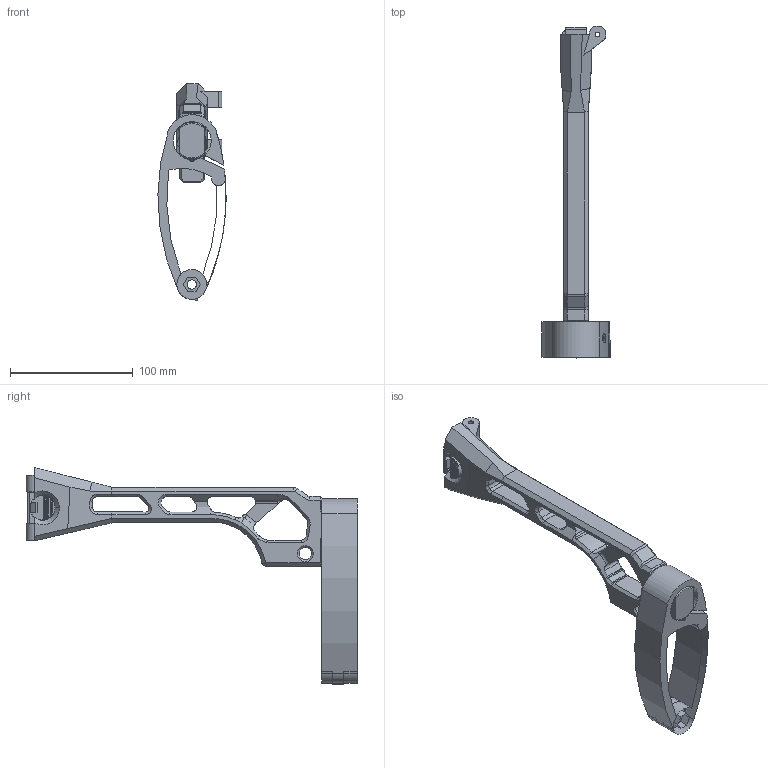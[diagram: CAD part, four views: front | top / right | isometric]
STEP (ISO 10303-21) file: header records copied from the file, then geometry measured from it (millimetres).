
FILE_DESCRIPTION(('STEP AP214'),'1');
FILE_NAME('IMA Scorpion Skeleton Stock with TH Brace (Vityaz Stock compatable).stp','2020-10-16T05:45:46',(' '),(' '),'Spatial InterOp 3D',' ',' ');
FILE_SCHEMA(('AUTOMOTIVE_DESIGN { 1 0 10303 214 1 1 1 1 }'));
Length unit declared in the file: metre
Products named in the file (6): IMA Scorpion Skeleton Stock with TH Brace (Vityaz Stock compatable); Component17; IMA Skeleton Brace (Vityaz Compatable); Tailhook ass; TailhookA; TailhookB
Assembly tree (5 placements, depth 3):
  IMA Scorpion Skeleton Stock with TH Brace (Vityaz Stock compatable)
    Component17
    IMA Skeleton Brace (Vityaz Compatable)
    Tailhook ass
      TailhookA
      TailhookB
Bounding box: 55.54 x 270.19 x 176.52 mm (x, y, z)
Volume: 237084.1 mm3; surface area: 71710.9 mm2
Topology: 4 solids, 4 shells, 413 faces, 1107 edges, 702 vertices
Faces by surface type: plane 216, cylinder 131, cone 56, torus 10
Entity records: 13890 total; most frequent: CARTESIAN_POINT 3208, DIRECTION 2237, ORIENTED_EDGE 2214, EDGE_CURVE 1107, AXIS2_PLACEMENT_3D 794, VERTEX_POINT 702, LINE 649, VECTOR 649
